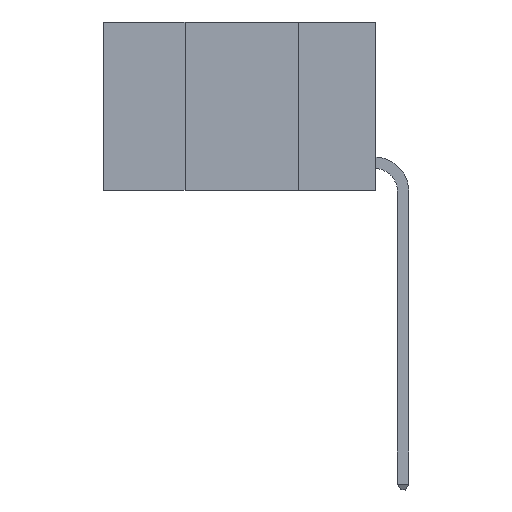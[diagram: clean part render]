
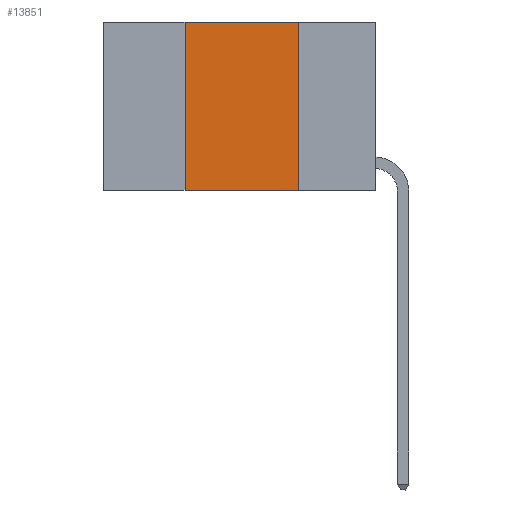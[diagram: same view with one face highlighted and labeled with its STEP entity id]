
A CAD part, left-side view. The second image highlights one B-rep face of the part: STEP entity #13851.
In plain terms, the highlighted planar face has unit normal (-1, 0, 0).
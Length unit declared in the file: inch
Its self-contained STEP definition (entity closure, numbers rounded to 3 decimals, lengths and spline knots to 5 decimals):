
#1519 = CARTESIAN_POINT ( 'NONE',  ( 0., 0.17, 0. ) ) ;
#2207 = VERTEX_POINT ( 'NONE', #15726 ) ;
#2312 = CARTESIAN_POINT ( 'NONE',  ( 0., 0.17, -0.37 ) ) ;
#2809 = VERTEX_POINT ( 'NONE', #4942 ) ;
#3103 = ORIENTED_EDGE ( 'NONE', *, *, #9658, .T. ) ;
#4942 = CARTESIAN_POINT ( 'NONE',  ( 0., 0.17, 0. ) ) ;
#5197 = EDGE_CURVE ( 'NONE', #2207, #2809, #6635, .T. ) ;
#5408 = CARTESIAN_POINT ( 'NONE',  ( 0., 0.6, -0.37 ) ) ;
#6236 = VECTOR ( 'NONE', #11962, 39.37008 ) ;
#6635 = LINE ( 'NONE', #7505, #16240 ) ;
#6672 = CARTESIAN_POINT ( 'NONE',  ( 0., 0.42, 0. ) ) ;
#6786 = VECTOR ( 'NONE', #8002, 39.37008 ) ;
#6998 = CARTESIAN_POINT ( 'NONE',  ( 0., 0.6, 0. ) ) ;
#7400 = EDGE_CURVE ( 'NONE', #13135, #2207, #16775, .T. ) ;
#7505 = CARTESIAN_POINT ( 'NONE',  ( 0., 0.6, 0. ) ) ;
#7701 = ORIENTED_EDGE ( 'NONE', *, *, #5197, .F. ) ;
#8002 = DIRECTION ( 'NONE',  ( 0., 0., 1. ) ) ;
#8027 = ORIENTED_EDGE ( 'NONE', *, *, #9729, .F. ) ;
#8329 = DIRECTION ( 'NONE',  ( 0., 0., -1. ) ) ;
#9584 = ORIENTED_EDGE ( 'NONE', *, *, #7400, .F. ) ;
#9658 = EDGE_CURVE ( 'NONE', #13135, #12345, #9713, .T. ) ;
#9713 = LINE ( 'NONE', #5408, #6236 ) ;
#9729 = EDGE_CURVE ( 'NONE', #2809, #12345, #15065, .T. ) ;
#10783 = CARTESIAN_POINT ( 'NONE',  ( 0., 0.42, -0.37 ) ) ;
#10864 = DIRECTION ( 'NONE',  ( 0., 0., -1. ) ) ;
#11962 = DIRECTION ( 'NONE',  ( 0., -1., 0. ) ) ;
#11989 = VECTOR ( 'NONE', #10864, 39.37008 ) ;
#12345 = VERTEX_POINT ( 'NONE', #2312 ) ;
#13135 = VERTEX_POINT ( 'NONE', #10783 ) ;
#13851 = ADVANCED_FACE ( 'NONE', ( #15110 ), #14898, .F. ) ;
#14291 = EDGE_LOOP ( 'NONE', ( #8027, #7701, #9584, #3103 ) ) ;
#14434 = AXIS2_PLACEMENT_3D ( 'NONE', #6998, #16139, #8329 ) ;
#14898 = PLANE ( 'NONE',  #14434 ) ;
#15065 = LINE ( 'NONE', #1519, #11989 ) ;
#15110 = FACE_OUTER_BOUND ( 'NONE', #14291, .T. ) ;
#15374 = DIRECTION ( 'NONE',  ( 0., -1., 0. ) ) ;
#15726 = CARTESIAN_POINT ( 'NONE',  ( 0., 0.42, 0. ) ) ;
#16139 = DIRECTION ( 'NONE',  ( 1., 0., 0. ) ) ;
#16240 = VECTOR ( 'NONE', #15374, 39.37008 ) ;
#16775 = LINE ( 'NONE', #6672, #6786 ) ;
